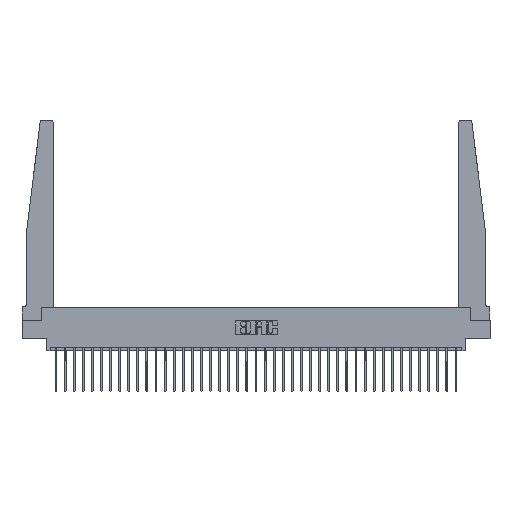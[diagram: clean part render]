
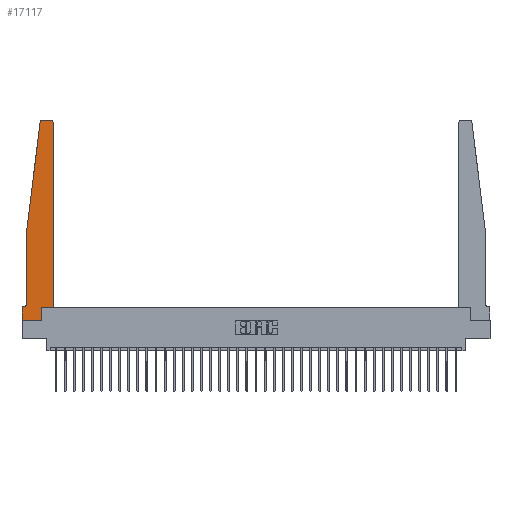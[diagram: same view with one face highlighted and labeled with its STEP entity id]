
A CAD part, top view. The second image highlights one B-rep face of the part: STEP entity #17117.
In plain terms, the highlighted planar face has unit normal (0, 0, 1).
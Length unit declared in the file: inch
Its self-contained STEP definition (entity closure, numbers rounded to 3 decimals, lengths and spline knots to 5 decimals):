
#92 = AXIS2_PLACEMENT_3D ( 'NONE', #210, #10818, #21385 ) ;
#205 = VERTEX_POINT ( 'NONE', #2580 ) ;
#210 = CARTESIAN_POINT ( 'NONE',  ( 0.015, 0.2375, 0.37 ) ) ;
#607 = AXIS2_PLACEMENT_3D ( 'NONE', #28477, #31441, #10079 ) ;
#1143 = VECTOR ( 'NONE', #4893, 39.37008 ) ;
#1317 = VERTEX_POINT ( 'NONE', #32096 ) ;
#1546 = VERTEX_POINT ( 'NONE', #19661 ) ;
#1594 = LINE ( 'NONE', #19818, #7693 ) ;
#1987 = ORIENTED_EDGE ( 'NONE', *, *, #24115, .T. ) ;
#2137 = VERTEX_POINT ( 'NONE', #27657 ) ;
#2580 = CARTESIAN_POINT ( 'NONE',  ( 0.27653, 2.75, 0.37 ) ) ;
#3596 = CARTESIAN_POINT ( 'NONE',  ( 0.425, 0.18, 0.37 ) ) ;
#3758 = CARTESIAN_POINT ( 'NONE',  ( 0.395, 2.75, 0.37 ) ) ;
#4893 = DIRECTION ( 'NONE',  ( -1., 0., 0. ) ) ;
#5035 = DIRECTION ( 'NONE',  ( -0.122, -0.992, 0. ) ) ;
#5288 = ORIENTED_EDGE ( 'NONE', *, *, #21713, .T. ) ;
#5438 = ORIENTED_EDGE ( 'NONE', *, *, #27641, .T. ) ;
#5980 = ORIENTED_EDGE ( 'NONE', *, *, #19603, .T. ) ;
#6304 = VECTOR ( 'NONE', #5035, 39.37008 ) ;
#7295 = EDGE_CURVE ( 'NONE', #1546, #23864, #7572, .T. ) ;
#7320 = CARTESIAN_POINT ( 'NONE',  ( 0.27653, 2.72, 0.37 ) ) ;
#7570 = DIRECTION ( 'NONE',  ( 0., -1., 0. ) ) ;
#7572 = LINE ( 'NONE', #26131, #33628 ) ;
#7693 = VECTOR ( 'NONE', #27806, 39.37008 ) ;
#8990 = ORIENTED_EDGE ( 'NONE', *, *, #12435, .T. ) ;
#9522 = CARTESIAN_POINT ( 'NONE',  ( 0., 0., 0.37 ) ) ;
#9732 = CARTESIAN_POINT ( 'NONE',  ( 0.425, 0.18, 0.37 ) ) ;
#10079 = DIRECTION ( 'NONE',  ( 1., 0., 0. ) ) ;
#10261 = CARTESIAN_POINT ( 'NONE',  ( 0.25, 2.75, 0.37 ) ) ;
#10343 = VERTEX_POINT ( 'NONE', #31032 ) ;
#10780 = LINE ( 'NONE', #10261, #1143 ) ;
#10818 = DIRECTION ( 'NONE',  ( 0., 0., -1. ) ) ;
#11556 = DIRECTION ( 'NONE',  ( 0., -1., 0. ) ) ;
#11725 = CARTESIAN_POINT ( 'NONE',  ( 0.395, 2.72, 0.37 ) ) ;
#12331 = PLANE ( 'NONE',  #607 ) ;
#12435 = EDGE_CURVE ( 'NONE', #2137, #15798, #1594, .T. ) ;
#12669 = FACE_OUTER_BOUND ( 'NONE', #24916, .T. ) ;
#12724 = ORIENTED_EDGE ( 'NONE', *, *, #18086, .T. ) ;
#12788 = ORIENTED_EDGE ( 'NONE', *, *, #28934, .T. ) ;
#12929 = VECTOR ( 'NONE', #7570, 39.37008 ) ;
#13176 = EDGE_CURVE ( 'NONE', #23864, #17035, #17247, .T. ) ;
#13978 = EDGE_CURVE ( 'NONE', #27586, #205, #10780, .T. ) ;
#14165 = DIRECTION ( 'NONE',  ( 0., 1., 0. ) ) ;
#15073 = CIRCLE ( 'NONE', #92, 0.05 ) ;
#15798 = VERTEX_POINT ( 'NONE', #18199 ) ;
#16572 = CARTESIAN_POINT ( 'NONE',  ( 0.425, 0.18, 0.37 ) ) ;
#16902 = VERTEX_POINT ( 'NONE', #19644 ) ;
#16921 = DIRECTION ( 'NONE',  ( 0., 0., 1. ) ) ;
#17035 = VERTEX_POINT ( 'NONE', #9732 ) ;
#17117 = ADVANCED_FACE ( 'NONE', ( #12669 ), #12331, .T. ) ;
#17247 = LINE ( 'NONE', #16572, #28241 ) ;
#17483 = DIRECTION ( 'NONE',  ( 1., 0., 0. ) ) ;
#18086 = EDGE_CURVE ( 'NONE', #10343, #2137, #15073, .T. ) ;
#18199 = CARTESIAN_POINT ( 'NONE',  ( 0., 0.1875, 0.37 ) ) ;
#18464 = CARTESIAN_POINT ( 'NONE',  ( 0., 0., 0.37 ) ) ;
#18536 = CIRCLE ( 'NONE', #22987, 0.03 ) ;
#18858 = CARTESIAN_POINT ( 'NONE',  ( 0.2605, 0.18, 0.37 ) ) ;
#19484 = VERTEX_POINT ( 'NONE', #23078 ) ;
#19538 = LINE ( 'NONE', #22464, #23090 ) ;
#19603 = EDGE_CURVE ( 'NONE', #19484, #22989, #26368, .T. ) ;
#19644 = CARTESIAN_POINT ( 'NONE',  ( 0., 0., 0.37 ) ) ;
#19661 = CARTESIAN_POINT ( 'NONE',  ( 0.2605, 0., 0.37 ) ) ;
#19818 = CARTESIAN_POINT ( 'NONE',  ( 0.065, 0.1875, 0.37 ) ) ;
#20177 = ORIENTED_EDGE ( 'NONE', *, *, #23440, .T. ) ;
#20390 = ORIENTED_EDGE ( 'NONE', *, *, #7295, .T. ) ;
#21162 = EDGE_CURVE ( 'NONE', #16902, #1546, #33326, .T. ) ;
#21385 = DIRECTION ( 'NONE',  ( -1., 0., 0. ) ) ;
#21713 = EDGE_CURVE ( 'NONE', #15798, #16902, #24044, .T. ) ;
#22464 = CARTESIAN_POINT ( 'NONE',  ( 0.065, 1.25, 0.37 ) ) ;
#22987 = AXIS2_PLACEMENT_3D ( 'NONE', #7320, #31432, #26207 ) ;
#22989 = VERTEX_POINT ( 'NONE', #25266 ) ;
#23078 = CARTESIAN_POINT ( 'NONE',  ( 0.24675, 2.72367, 0.37 ) ) ;
#23090 = VECTOR ( 'NONE', #11556, 39.37008 ) ;
#23440 = EDGE_CURVE ( 'NONE', #205, #19484, #18536, .T. ) ;
#23701 = DIRECTION ( 'NONE',  ( 0., 1., 0. ) ) ;
#23864 = VERTEX_POINT ( 'NONE', #18858 ) ;
#24044 = LINE ( 'NONE', #18464, #12929 ) ;
#24115 = EDGE_CURVE ( 'NONE', #17035, #1317, #30333, .T. ) ;
#24916 = EDGE_LOOP ( 'NONE', ( #29601, #20177, #5980, #5438, #12724, #8990, #5288, #29414, #20390, #34089, #1987, #12788 ) ) ;
#25225 = VECTOR ( 'NONE', #14165, 39.37008 ) ;
#25266 = CARTESIAN_POINT ( 'NONE',  ( 0.065, 1.25, 0.37 ) ) ;
#26131 = CARTESIAN_POINT ( 'NONE',  ( 0.2605, 0.18, 0.37 ) ) ;
#26207 = DIRECTION ( 'NONE',  ( 1., 0., 0. ) ) ;
#26368 = LINE ( 'NONE', #28804, #6304 ) ;
#27190 = DIRECTION ( 'NONE',  ( 1., 0., 0. ) ) ;
#27586 = VERTEX_POINT ( 'NONE', #3758 ) ;
#27641 = EDGE_CURVE ( 'NONE', #22989, #10343, #19538, .T. ) ;
#27657 = CARTESIAN_POINT ( 'NONE',  ( 0.015, 0.1875, 0.37 ) ) ;
#27693 = DIRECTION ( 'NONE',  ( 1., 0., 0. ) ) ;
#27806 = DIRECTION ( 'NONE',  ( -1., 0., 0. ) ) ;
#28241 = VECTOR ( 'NONE', #27190, 39.37008 ) ;
#28451 = VECTOR ( 'NONE', #17483, 39.37008 ) ;
#28477 = CARTESIAN_POINT ( 'NONE',  ( 0., 0.1875, 0.37 ) ) ;
#28804 = CARTESIAN_POINT ( 'NONE',  ( 0.065, 1.25, 0.37 ) ) ;
#28934 = EDGE_CURVE ( 'NONE', #1317, #27586, #30933, .T. ) ;
#29414 = ORIENTED_EDGE ( 'NONE', *, *, #21162, .T. ) ;
#29601 = ORIENTED_EDGE ( 'NONE', *, *, #13978, .T. ) ;
#30333 = LINE ( 'NONE', #3596, #25225 ) ;
#30933 = CIRCLE ( 'NONE', #34238, 0.03 ) ;
#31032 = CARTESIAN_POINT ( 'NONE',  ( 0.065, 0.2375, 0.37 ) ) ;
#31432 = DIRECTION ( 'NONE',  ( 0., 0., 1. ) ) ;
#31441 = DIRECTION ( 'NONE',  ( 0., 0., 1. ) ) ;
#32096 = CARTESIAN_POINT ( 'NONE',  ( 0.425, 2.72, 0.37 ) ) ;
#33326 = LINE ( 'NONE', #9522, #28451 ) ;
#33628 = VECTOR ( 'NONE', #23701, 39.37008 ) ;
#34089 = ORIENTED_EDGE ( 'NONE', *, *, #13176, .T. ) ;
#34238 = AXIS2_PLACEMENT_3D ( 'NONE', #11725, #16921, #27693 ) ;
